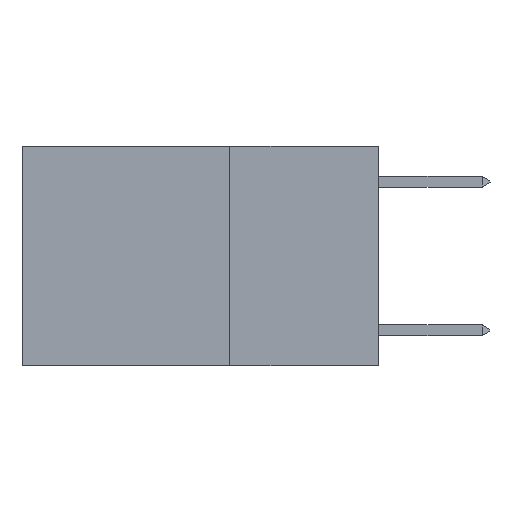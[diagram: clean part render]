
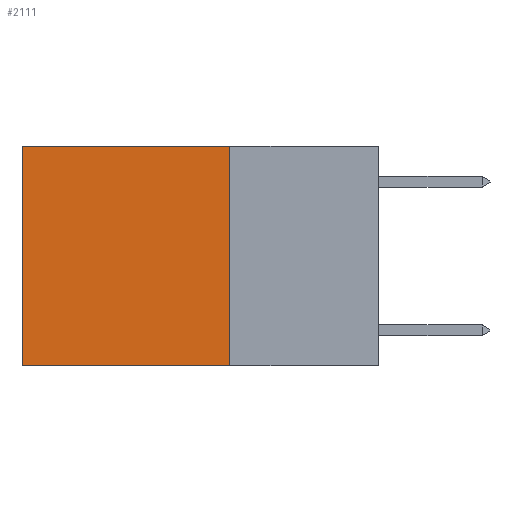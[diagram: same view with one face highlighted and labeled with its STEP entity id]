
A CAD part, left-side view. The second image highlights one B-rep face of the part: STEP entity #2111.
In plain terms, the highlighted planar face has unit normal (-1, 0, 0).
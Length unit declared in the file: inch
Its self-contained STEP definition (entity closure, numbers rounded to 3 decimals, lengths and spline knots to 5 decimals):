
#102 = DIRECTION ( 'NONE',  ( 0., 1., 0. ) ) ;
#831 = CARTESIAN_POINT ( 'NONE',  ( 0.2625, 0.25, -0.37 ) ) ;
#914 = VERTEX_POINT ( 'NONE', #11985 ) ;
#1138 = DIRECTION ( 'NONE',  ( 1., 0., 0. ) ) ;
#1580 = ORIENTED_EDGE ( 'NONE', *, *, #6554, .T. ) ;
#1728 = EDGE_CURVE ( 'NONE', #914, #3796, #11144, .T. ) ;
#1884 = VECTOR ( 'NONE', #12226, 39.37008 ) ;
#2025 = CARTESIAN_POINT ( 'NONE',  ( 0.2625, 0.25, 0. ) ) ;
#2111 = ADVANCED_FACE ( 'NONE', ( #4738 ), #10877, .F. ) ;
#2263 = DIRECTION ( 'NONE',  ( 0., 0., -1. ) ) ;
#2559 = EDGE_CURVE ( 'NONE', #914, #3603, #11177, .T. ) ;
#3048 = VECTOR ( 'NONE', #102, 39.37008 ) ;
#3603 = VERTEX_POINT ( 'NONE', #11158 ) ;
#3796 = VERTEX_POINT ( 'NONE', #831 ) ;
#3910 = CARTESIAN_POINT ( 'NONE',  ( 0.2625, 0.6, -0.37 ) ) ;
#4065 = EDGE_CURVE ( 'NONE', #3796, #10096, #11341, .T. ) ;
#4148 = CARTESIAN_POINT ( 'NONE',  ( 0.2625, 0.25, -0.37 ) ) ;
#4738 = FACE_OUTER_BOUND ( 'NONE', #8944, .T. ) ;
#5420 = ORIENTED_EDGE ( 'NONE', *, *, #2559, .T. ) ;
#6554 = EDGE_CURVE ( 'NONE', #3603, #10096, #8553, .T. ) ;
#7877 = CARTESIAN_POINT ( 'NONE',  ( 0.2625, 0.25, 0. ) ) ;
#8137 = CARTESIAN_POINT ( 'NONE',  ( 0.2625, 0.25, 0. ) ) ;
#8426 = DIRECTION ( 'NONE',  ( 0., 0., -1. ) ) ;
#8553 = LINE ( 'NONE', #12649, #8568 ) ;
#8568 = VECTOR ( 'NONE', #8426, 39.37008 ) ;
#8944 = EDGE_LOOP ( 'NONE', ( #1580, #11196, #9617, #5420 ) ) ;
#9617 = ORIENTED_EDGE ( 'NONE', *, *, #1728, .F. ) ;
#10096 = VERTEX_POINT ( 'NONE', #3910 ) ;
#10365 = AXIS2_PLACEMENT_3D ( 'NONE', #7877, #1138, #2263 ) ;
#10877 = PLANE ( 'NONE',  #10365 ) ;
#11144 = LINE ( 'NONE', #8137, #1884 ) ;
#11158 = CARTESIAN_POINT ( 'NONE',  ( 0.2625, 0.6, 0. ) ) ;
#11177 = LINE ( 'NONE', #2025, #3048 ) ;
#11196 = ORIENTED_EDGE ( 'NONE', *, *, #4065, .F. ) ;
#11341 = LINE ( 'NONE', #4148, #12797 ) ;
#11985 = CARTESIAN_POINT ( 'NONE',  ( 0.2625, 0.25, 0. ) ) ;
#12226 = DIRECTION ( 'NONE',  ( 0., 0., -1. ) ) ;
#12306 = DIRECTION ( 'NONE',  ( 0., 1., 0. ) ) ;
#12649 = CARTESIAN_POINT ( 'NONE',  ( 0.2625, 0.6, 0. ) ) ;
#12797 = VECTOR ( 'NONE', #12306, 39.37008 ) ;
